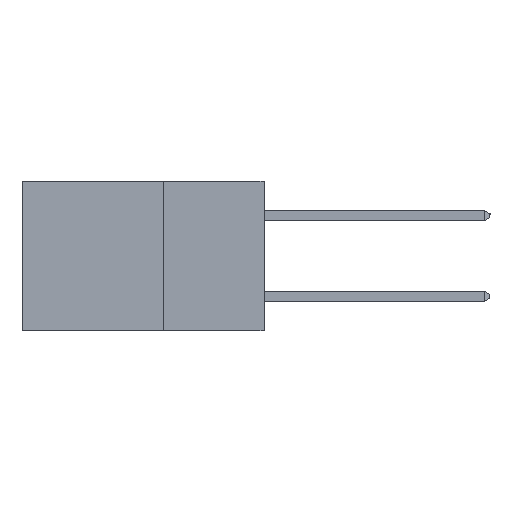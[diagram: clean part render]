
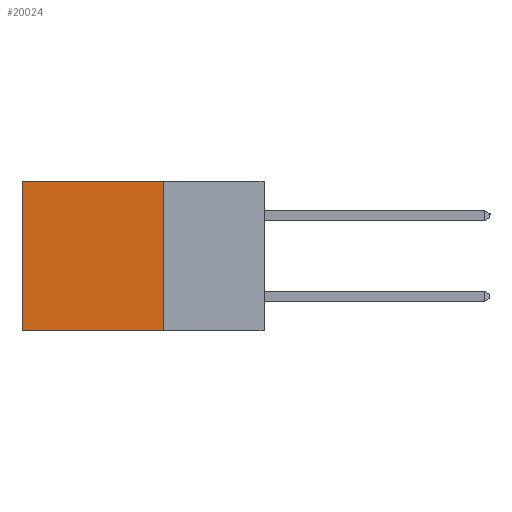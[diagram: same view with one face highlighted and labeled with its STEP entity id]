
A CAD part, left-side view. The second image highlights one B-rep face of the part: STEP entity #20024.
In plain terms, the highlighted planar face has unit normal (-1, 0, 0).
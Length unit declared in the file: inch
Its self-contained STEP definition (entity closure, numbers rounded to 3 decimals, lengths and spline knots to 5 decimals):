
#1210 = DIRECTION ( 'NONE',  ( 0., 0., -1. ) ) ;
#1437 = VECTOR ( 'NONE', #8859, 39.37008 ) ;
#1741 = CARTESIAN_POINT ( 'NONE',  ( 0.2615, 0.25, -0.37 ) ) ;
#1777 = DIRECTION ( 'NONE',  ( 0., 1., 0. ) ) ;
#2849 = CARTESIAN_POINT ( 'NONE',  ( 0.2615, 0.25, -0.37 ) ) ;
#3153 = EDGE_CURVE ( 'NONE', #16953, #17020, #12760, .T. ) ;
#3395 = CARTESIAN_POINT ( 'NONE',  ( 0.2615, 0.6, 0. ) ) ;
#3762 = VECTOR ( 'NONE', #1210, 39.37008 ) ;
#5210 = CARTESIAN_POINT ( 'NONE',  ( 0.2615, 0.25, 0. ) ) ;
#6983 = DIRECTION ( 'NONE',  ( 0., 1., 0. ) ) ;
#7109 = AXIS2_PLACEMENT_3D ( 'NONE', #18804, #10136, #8258 ) ;
#7338 = CARTESIAN_POINT ( 'NONE',  ( 0.2615, 0.6, -0.37 ) ) ;
#7919 = VERTEX_POINT ( 'NONE', #17855 ) ;
#8258 = DIRECTION ( 'NONE',  ( 0., 0., -1. ) ) ;
#8859 = DIRECTION ( 'NONE',  ( 0., 0., -1. ) ) ;
#9844 = ORIENTED_EDGE ( 'NONE', *, *, #3153, .T. ) ;
#10136 = DIRECTION ( 'NONE',  ( 1., 0., 0. ) ) ;
#10176 = VERTEX_POINT ( 'NONE', #1741 ) ;
#10557 = ORIENTED_EDGE ( 'NONE', *, *, #14579, .T. ) ;
#10710 = ORIENTED_EDGE ( 'NONE', *, *, #15563, .F. ) ;
#10724 = LINE ( 'NONE', #2849, #3762 ) ;
#11143 = LINE ( 'NONE', #5210, #20193 ) ;
#12460 = VECTOR ( 'NONE', #1777, 39.37008 ) ;
#12760 = LINE ( 'NONE', #21010, #1437 ) ;
#14526 = ORIENTED_EDGE ( 'NONE', *, *, #15253, .F. ) ;
#14579 = EDGE_CURVE ( 'NONE', #7919, #16953, #11143, .T. ) ;
#14585 = FACE_OUTER_BOUND ( 'NONE', #16578, .T. ) ;
#15253 = EDGE_CURVE ( 'NONE', #10176, #17020, #20320, .T. ) ;
#15563 = EDGE_CURVE ( 'NONE', #7919, #10176, #10724, .T. ) ;
#16388 = CARTESIAN_POINT ( 'NONE',  ( 0.2615, 0.25, -0.37 ) ) ;
#16578 = EDGE_LOOP ( 'NONE', ( #9844, #14526, #10710, #10557 ) ) ;
#16953 = VERTEX_POINT ( 'NONE', #3395 ) ;
#17020 = VERTEX_POINT ( 'NONE', #7338 ) ;
#17855 = CARTESIAN_POINT ( 'NONE',  ( 0.2615, 0.25, 0. ) ) ;
#18804 = CARTESIAN_POINT ( 'NONE',  ( 0.2615, 0.25, -0.37 ) ) ;
#20024 = ADVANCED_FACE ( 'NONE', ( #14585 ), #22986, .F. ) ;
#20193 = VECTOR ( 'NONE', #6983, 39.37008 ) ;
#20320 = LINE ( 'NONE', #16388, #12460 ) ;
#21010 = CARTESIAN_POINT ( 'NONE',  ( 0.2615, 0.6, -0.37 ) ) ;
#22986 = PLANE ( 'NONE',  #7109 ) ;
